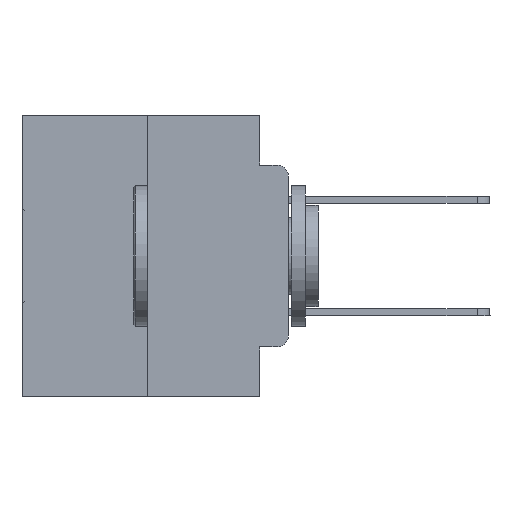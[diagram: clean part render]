
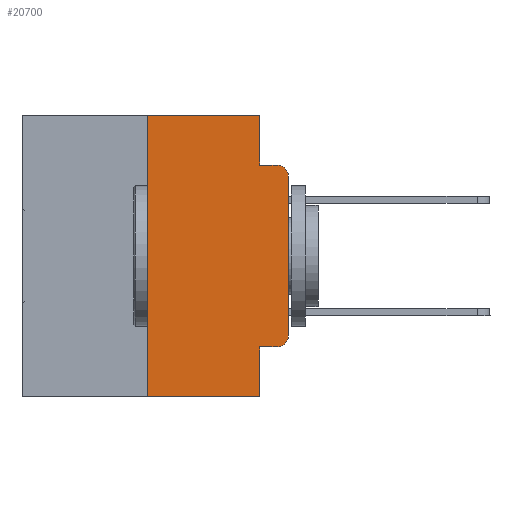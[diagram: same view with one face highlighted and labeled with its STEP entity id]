
A CAD part, left-side view. The second image highlights one B-rep face of the part: STEP entity #20700.
In plain terms, the highlighted planar face has unit normal (-1, 0, 0).
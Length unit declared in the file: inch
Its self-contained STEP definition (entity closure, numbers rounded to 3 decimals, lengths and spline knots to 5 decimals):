
#77 = CARTESIAN_POINT ( 'NONE',  ( 0., 0.051, -0.5 ) ) ;
#199 = EDGE_CURVE ( 'NONE', #11727, #5140, #19277, .T. ) ;
#791 = VERTEX_POINT ( 'NONE', #14520 ) ;
#1315 = CARTESIAN_POINT ( 'NONE',  ( 0., 0.02, -0.3915 ) ) ;
#1528 = DIRECTION ( 'NONE',  ( -1., 0., 0. ) ) ;
#2515 = AXIS2_PLACEMENT_3D ( 'NONE', #1315, #1528, #18324 ) ;
#2758 = ORIENTED_EDGE ( 'NONE', *, *, #15150, .F. ) ;
#3144 = CARTESIAN_POINT ( 'NONE',  ( 0., 0.051, -0.0885 ) ) ;
#3250 = DIRECTION ( 'NONE',  ( 0., -1., 0. ) ) ;
#3355 = DIRECTION ( 'NONE',  ( 1., 0., 0. ) ) ;
#3910 = VERTEX_POINT ( 'NONE', #77 ) ;
#4060 = DIRECTION ( 'NONE',  ( 0., -1., 0. ) ) ;
#4258 = CARTESIAN_POINT ( 'NONE',  ( 0., 0.051, 0. ) ) ;
#4690 = CARTESIAN_POINT ( 'NONE',  ( 0., 0.051, -0.0885 ) ) ;
#4879 = FACE_OUTER_BOUND ( 'NONE', #27017, .T. ) ;
#5140 = VERTEX_POINT ( 'NONE', #12166 ) ;
#5148 = ORIENTED_EDGE ( 'NONE', *, *, #199, .T. ) ;
#5543 = VECTOR ( 'NONE', #4060, 39.37008 ) ;
#6016 = CARTESIAN_POINT ( 'NONE',  ( 0., 0.051, -0.4115 ) ) ;
#6561 = DIRECTION ( 'NONE',  ( 0., -1., 0. ) ) ;
#6955 = VERTEX_POINT ( 'NONE', #25022 ) ;
#7718 = CARTESIAN_POINT ( 'NONE',  ( 0., 0.051, -0.4115 ) ) ;
#8238 = VECTOR ( 'NONE', #14620, 39.37008 ) ;
#8547 = LINE ( 'NONE', #19161, #26091 ) ;
#8901 = DIRECTION ( 'NONE',  ( 0., 0., 1. ) ) ;
#9389 = DIRECTION ( 'NONE',  ( 0., 0., 1. ) ) ;
#9438 = CARTESIAN_POINT ( 'NONE',  ( 0., 0., -0.1085 ) ) ;
#9505 = VECTOR ( 'NONE', #20072, 39.37008 ) ;
#10424 = AXIS2_PLACEMENT_3D ( 'NONE', #27929, #3355, #20372 ) ;
#11447 = VERTEX_POINT ( 'NONE', #4690 ) ;
#11597 = ORIENTED_EDGE ( 'NONE', *, *, #23010, .F. ) ;
#11727 = VERTEX_POINT ( 'NONE', #9438 ) ;
#11739 = AXIS2_PLACEMENT_3D ( 'NONE', #28723, #14171, #31156 ) ;
#12166 = CARTESIAN_POINT ( 'NONE',  ( 0., 0.02, -0.0885 ) ) ;
#12479 = CIRCLE ( 'NONE', #2515, 0.02 ) ;
#12480 = CARTESIAN_POINT ( 'NONE',  ( 0., 0.25, -0.5 ) ) ;
#12536 = EDGE_CURVE ( 'NONE', #6955, #24409, #21927, .T. ) ;
#12538 = EDGE_CURVE ( 'NONE', #791, #24777, #12479, .T. ) ;
#13382 = CARTESIAN_POINT ( 'NONE',  ( 0., 0.25, 0. ) ) ;
#13681 = LINE ( 'NONE', #30644, #15560 ) ;
#13682 = EDGE_CURVE ( 'NONE', #24641, #3910, #13681, .T. ) ;
#13925 = ORIENTED_EDGE ( 'NONE', *, *, #13682, .T. ) ;
#14171 = DIRECTION ( 'NONE',  ( -1., 0., 0. ) ) ;
#14520 = CARTESIAN_POINT ( 'NONE',  ( 0., 0.02, -0.4115 ) ) ;
#14620 = DIRECTION ( 'NONE',  ( 0., 0., -1. ) ) ;
#15150 = EDGE_CURVE ( 'NONE', #16263, #3910, #19302, .T. ) ;
#15501 = ORIENTED_EDGE ( 'NONE', *, *, #16199, .T. ) ;
#15560 = VECTOR ( 'NONE', #6561, 39.37008 ) ;
#16199 = EDGE_CURVE ( 'NONE', #24777, #11727, #8547, .T. ) ;
#16263 = VERTEX_POINT ( 'NONE', #6016 ) ;
#16647 = ORIENTED_EDGE ( 'NONE', *, *, #12538, .T. ) ;
#17516 = LINE ( 'NONE', #3144, #21681 ) ;
#17737 = PLANE ( 'NONE',  #10424 ) ;
#18324 = DIRECTION ( 'NONE',  ( 0., 0., -1. ) ) ;
#18642 = CARTESIAN_POINT ( 'NONE',  ( 0., 0.473, 0. ) ) ;
#18708 = DIRECTION ( 'NONE',  ( 0., 0., -1. ) ) ;
#19161 = CARTESIAN_POINT ( 'NONE',  ( 0., 0., 0. ) ) ;
#19277 = CIRCLE ( 'NONE', #11739, 0.02 ) ;
#19302 = LINE ( 'NONE', #29182, #8238 ) ;
#19489 = EDGE_CURVE ( 'NONE', #11447, #5140, #17516, .T. ) ;
#20072 = DIRECTION ( 'NONE',  ( 0., -1., 0. ) ) ;
#20087 = ORIENTED_EDGE ( 'NONE', *, *, #19489, .F. ) ;
#20372 = DIRECTION ( 'NONE',  ( 0., 0., -1. ) ) ;
#20700 = ADVANCED_FACE ( 'NONE', ( #4879 ), #17737, .F. ) ;
#21040 = CARTESIAN_POINT ( 'NONE',  ( 0., 0.051, 0. ) ) ;
#21326 = VECTOR ( 'NONE', #8901, 39.37008 ) ;
#21473 = VECTOR ( 'NONE', #18708, 39.37008 ) ;
#21681 = VECTOR ( 'NONE', #3250, 39.37008 ) ;
#21927 = LINE ( 'NONE', #18642, #5543 ) ;
#22452 = ORIENTED_EDGE ( 'NONE', *, *, #26583, .T. ) ;
#23010 = EDGE_CURVE ( 'NONE', #24409, #11447, #25652, .T. ) ;
#23322 = CARTESIAN_POINT ( 'NONE',  ( 0., 0., -0.3915 ) ) ;
#24409 = VERTEX_POINT ( 'NONE', #4258 ) ;
#24641 = VERTEX_POINT ( 'NONE', #12480 ) ;
#24777 = VERTEX_POINT ( 'NONE', #23322 ) ;
#25022 = CARTESIAN_POINT ( 'NONE',  ( 0., 0.25, 0. ) ) ;
#25091 = ORIENTED_EDGE ( 'NONE', *, *, #26916, .F. ) ;
#25652 = LINE ( 'NONE', #21040, #21473 ) ;
#26091 = VECTOR ( 'NONE', #9389, 39.37008 ) ;
#26583 = EDGE_CURVE ( 'NONE', #16263, #791, #27011, .T. ) ;
#26916 = EDGE_CURVE ( 'NONE', #24641, #6955, #27803, .T. ) ;
#27011 = LINE ( 'NONE', #7718, #9505 ) ;
#27017 = EDGE_LOOP ( 'NONE', ( #15501, #5148, #20087, #11597, #31104, #25091, #13925, #2758, #22452, #16647 ) ) ;
#27803 = LINE ( 'NONE', #13382, #21326 ) ;
#27929 = CARTESIAN_POINT ( 'NONE',  ( 0., 0.473, 0. ) ) ;
#28723 = CARTESIAN_POINT ( 'NONE',  ( 0., 0.02, -0.1085 ) ) ;
#29182 = CARTESIAN_POINT ( 'NONE',  ( 0., 0.051, 0. ) ) ;
#30644 = CARTESIAN_POINT ( 'NONE',  ( 0., 0.473, -0.5 ) ) ;
#31104 = ORIENTED_EDGE ( 'NONE', *, *, #12536, .F. ) ;
#31156 = DIRECTION ( 'NONE',  ( 0., 0., -1. ) ) ;
